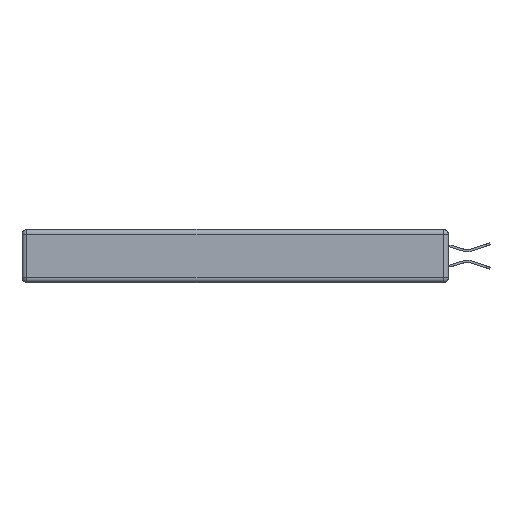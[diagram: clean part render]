
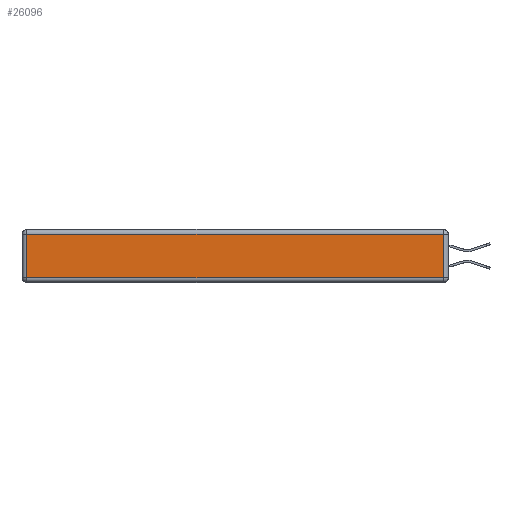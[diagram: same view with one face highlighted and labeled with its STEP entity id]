
A CAD part, left-side view. The second image highlights one B-rep face of the part: STEP entity #26096.
In plain terms, the highlighted planar face has unit normal (-1, 0, 0).
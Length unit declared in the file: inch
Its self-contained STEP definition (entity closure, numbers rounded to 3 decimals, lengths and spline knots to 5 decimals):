
#489 = VECTOR ( 'NONE', #9818, 39.37008 ) ;
#649 = CARTESIAN_POINT ( 'NONE',  ( 0., 0., -0.313 ) ) ;
#672 = PLANE ( 'NONE',  #13252 ) ;
#704 = CARTESIAN_POINT ( 'NONE',  ( 0., 2.72, -0.343 ) ) ;
#3325 = ORIENTED_EDGE ( 'NONE', *, *, #12494, .T. ) ;
#3890 = CARTESIAN_POINT ( 'NONE',  ( 0., 0.03, -0.03 ) ) ;
#4179 = VERTEX_POINT ( 'NONE', #3890 ) ;
#4359 = LINE ( 'NONE', #10282, #11093 ) ;
#8796 = VERTEX_POINT ( 'NONE', #24531 ) ;
#9818 = DIRECTION ( 'NONE',  ( 0., 0., -1. ) ) ;
#10158 = DIRECTION ( 'NONE',  ( 0., -1., 0. ) ) ;
#10282 = CARTESIAN_POINT ( 'NONE',  ( 0., 2.75, -0.03 ) ) ;
#11093 = VECTOR ( 'NONE', #12569, 39.37008 ) ;
#11271 = EDGE_CURVE ( 'NONE', #8796, #4179, #19167, .T. ) ;
#11741 = FACE_OUTER_BOUND ( 'NONE', #19973, .T. ) ;
#12494 = EDGE_CURVE ( 'NONE', #17242, #16633, #23370, .T. ) ;
#12569 = DIRECTION ( 'NONE',  ( 0., 1., 0. ) ) ;
#13252 = AXIS2_PLACEMENT_3D ( 'NONE', #14560, #18969, #19074 ) ;
#14560 = CARTESIAN_POINT ( 'NONE',  ( 0., 0., -0.343 ) ) ;
#15015 = ORIENTED_EDGE ( 'NONE', *, *, #23852, .T. ) ;
#15113 = LINE ( 'NONE', #649, #20481 ) ;
#16633 = VERTEX_POINT ( 'NONE', #27002 ) ;
#17242 = VERTEX_POINT ( 'NONE', #18622 ) ;
#17614 = CARTESIAN_POINT ( 'NONE',  ( 0., 0.03, -0.343 ) ) ;
#18622 = CARTESIAN_POINT ( 'NONE',  ( 0., 2.72, -0.03 ) ) ;
#18969 = DIRECTION ( 'NONE',  ( -1., 0., 0. ) ) ;
#19074 = DIRECTION ( 'NONE',  ( 0., 0., 1. ) ) ;
#19167 = LINE ( 'NONE', #17614, #23091 ) ;
#19973 = EDGE_LOOP ( 'NONE', ( #15015, #20426, #26999, #3325 ) ) ;
#20426 = ORIENTED_EDGE ( 'NONE', *, *, #11271, .T. ) ;
#20481 = VECTOR ( 'NONE', #10158, 39.37008 ) ;
#22502 = EDGE_CURVE ( 'NONE', #4179, #17242, #4359, .T. ) ;
#23091 = VECTOR ( 'NONE', #29436, 39.37008 ) ;
#23370 = LINE ( 'NONE', #704, #489 ) ;
#23852 = EDGE_CURVE ( 'NONE', #16633, #8796, #15113, .T. ) ;
#24531 = CARTESIAN_POINT ( 'NONE',  ( 0., 0.03, -0.313 ) ) ;
#26096 = ADVANCED_FACE ( 'NONE', ( #11741 ), #672, .T. ) ;
#26999 = ORIENTED_EDGE ( 'NONE', *, *, #22502, .T. ) ;
#27002 = CARTESIAN_POINT ( 'NONE',  ( 0., 2.72, -0.313 ) ) ;
#29436 = DIRECTION ( 'NONE',  ( 0., 0., 1. ) ) ;
